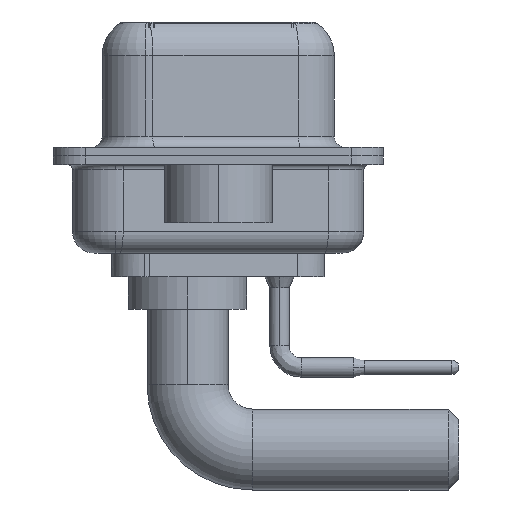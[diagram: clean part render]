
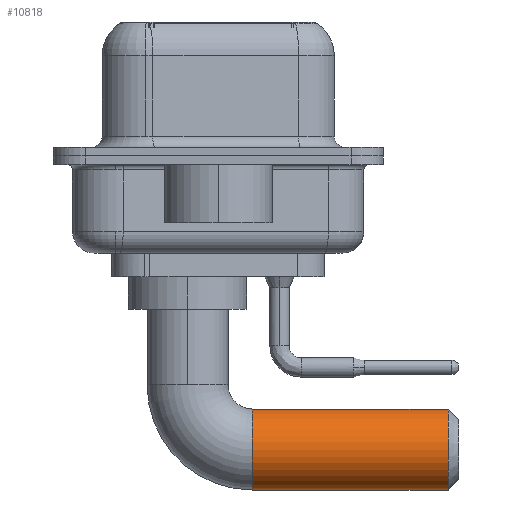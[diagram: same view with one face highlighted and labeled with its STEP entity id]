
A CAD part, left-side view. The second image highlights one B-rep face of the part: STEP entity #10818.
In plain terms, the highlighted cylindrical face has radius 1.875 mm (diameter 3.75 mm), a partial arc.
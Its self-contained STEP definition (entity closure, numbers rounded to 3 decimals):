
#29 = AXIS2_PLACEMENT_3D ( 'NONE', #11237, #9492, #6254 ) ;
#264 = DIRECTION ( 'NONE',  ( -1., 0., 0. ) ) ;
#1078 = DIRECTION ( 'NONE',  ( 0., 1., 0. ) ) ;
#1103 = VERTEX_POINT ( 'NONE', #7151 ) ;
#1241 = CARTESIAN_POINT ( 'NONE',  ( 0., -12.07, -4.625 ) ) ;
#2199 = DIRECTION ( 'NONE',  ( 0., -1., 0. ) ) ;
#2384 = CARTESIAN_POINT ( 'NONE',  ( 0., -3., -8.375 ) ) ;
#2687 = EDGE_CURVE ( 'NONE', #14454, #5346, #10220, .T. ) ;
#3390 = ORIENTED_EDGE ( 'NONE', *, *, #2687, .T. ) ;
#5274 = DIRECTION ( 'NONE',  ( 0., -1., 0. ) ) ;
#5340 = CARTESIAN_POINT ( 'NONE',  ( 0., -3., -4.625 ) ) ;
#5346 = VERTEX_POINT ( 'NONE', #9544 ) ;
#6231 = AXIS2_PLACEMENT_3D ( 'NONE', #16823, #2199, #264 ) ;
#6254 = DIRECTION ( 'NONE',  ( 0., 0., -1. ) ) ;
#7151 = CARTESIAN_POINT ( 'NONE',  ( 0., -3., -4.625 ) ) ;
#7554 = VECTOR ( 'NONE', #5274, 1000. ) ;
#9492 = DIRECTION ( 'NONE',  ( 0., -1., 0. ) ) ;
#9544 = CARTESIAN_POINT ( 'NONE',  ( 0., -12.07, -8.375 ) ) ;
#10220 = LINE ( 'NONE', #2384, #7554 ) ;
#10318 = ORIENTED_EDGE ( 'NONE', *, *, #14377, .T. ) ;
#10818 = ADVANCED_FACE ( 'NONE', ( #15767 ), #11129, .T. ) ;
#10842 = VERTEX_POINT ( 'NONE', #1241 ) ;
#11075 = CARTESIAN_POINT ( 'NONE',  ( 0., -12.07, -6.5 ) ) ;
#11129 = CYLINDRICAL_SURFACE ( 'NONE', #29, 1.875 ) ;
#11237 = CARTESIAN_POINT ( 'NONE',  ( 0., -3., -6.5 ) ) ;
#11911 = DIRECTION ( 'NONE',  ( 0., -1., 0. ) ) ;
#12084 = VECTOR ( 'NONE', #11911, 1000. ) ;
#12212 = EDGE_CURVE ( 'NONE', #1103, #10842, #20102, .T. ) ;
#13274 = EDGE_CURVE ( 'NONE', #5346, #10842, #17629, .T. ) ;
#13452 = ORIENTED_EDGE ( 'NONE', *, *, #13274, .T. ) ;
#14377 = EDGE_CURVE ( 'NONE', #1103, #14454, #15555, .T. ) ;
#14454 = VERTEX_POINT ( 'NONE', #15004 ) ;
#14541 = EDGE_LOOP ( 'NONE', ( #19172, #10318, #3390, #13452 ) ) ;
#15004 = CARTESIAN_POINT ( 'NONE',  ( 0., -3., -8.375 ) ) ;
#15234 = AXIS2_PLACEMENT_3D ( 'NONE', #11075, #1078, #15714 ) ;
#15555 = CIRCLE ( 'NONE', #6231, 1.875 ) ;
#15714 = DIRECTION ( 'NONE',  ( 0., 0., -1. ) ) ;
#15767 = FACE_OUTER_BOUND ( 'NONE', #14541, .T. ) ;
#16823 = CARTESIAN_POINT ( 'NONE',  ( 0., -3., -6.5 ) ) ;
#17629 = CIRCLE ( 'NONE', #15234, 1.875 ) ;
#19172 = ORIENTED_EDGE ( 'NONE', *, *, #12212, .F. ) ;
#20102 = LINE ( 'NONE', #5340, #12084 ) ;
